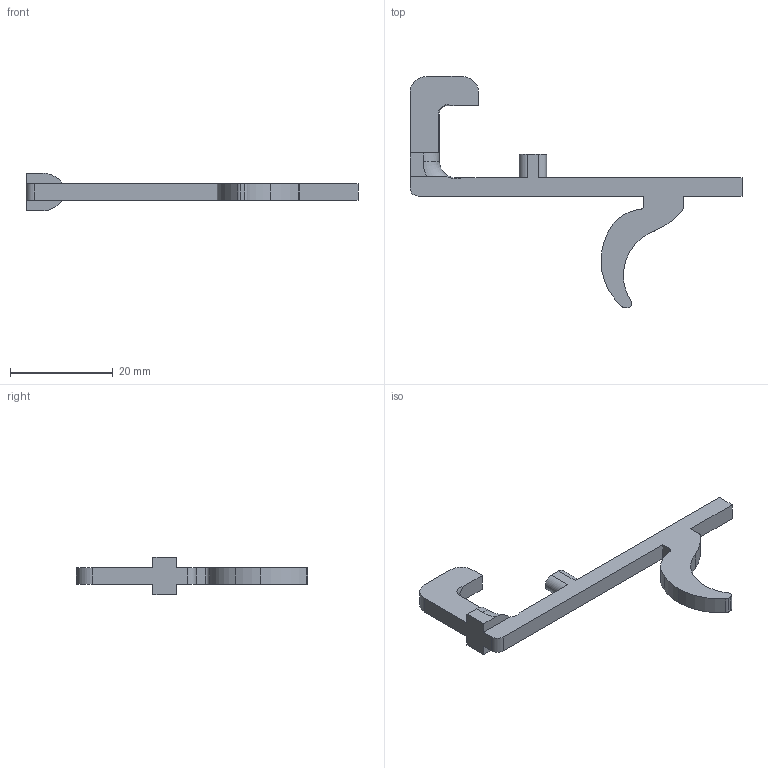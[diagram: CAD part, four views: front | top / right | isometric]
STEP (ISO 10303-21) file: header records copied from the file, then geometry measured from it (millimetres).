
FILE_DESCRIPTION (( 'STEP AP214' ), '1' );
FILE_NAME ('trigger.STEP', '2013-05-27T22:40:51', ( 'Asher' ), ( '' ), 'SwSTEP 2.0', 'SolidWorks 2013', '' );
FILE_SCHEMA (( 'AUTOMOTIVE_DESIGN' ));
Length unit declared in the file: millimetre
Products named in the file (1): trigger
Bounding box: 64.52 x 44.91 x 7.37 mm (x, y, z)
Volume: 1858.9 mm3; surface area: 1931.3 mm2
Topology: 1 solids, 1 shells, 48 faces, 134 edges, 88 vertices
Faces by surface type: plane 24, cylinder 20, torus 4
Entity records: 1606 total; most frequent: CARTESIAN_POINT 301, DIRECTION 274, ORIENTED_EDGE 268, EDGE_CURVE 134, AXIS2_PLACEMENT_3D 97, VERTEX_POINT 88, LINE 80, VECTOR 80
